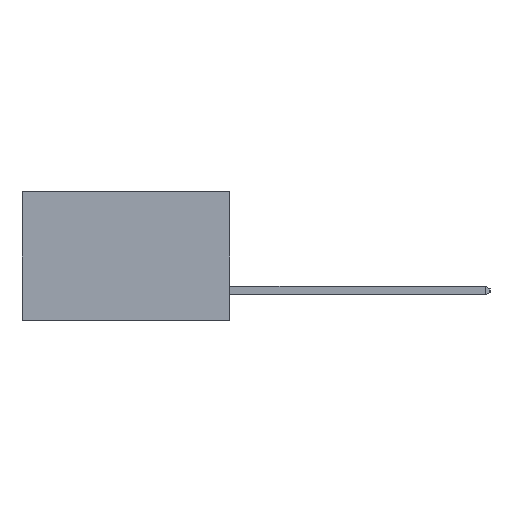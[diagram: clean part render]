
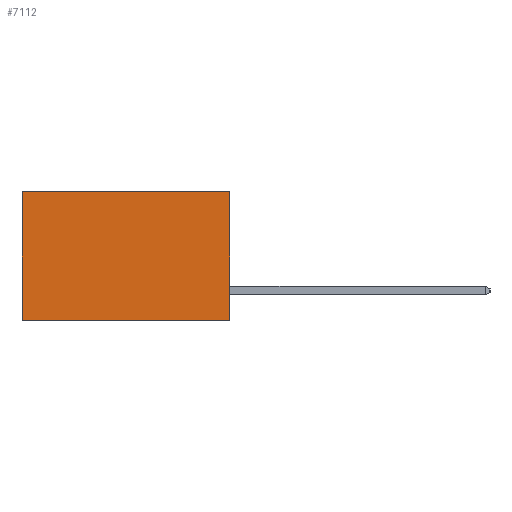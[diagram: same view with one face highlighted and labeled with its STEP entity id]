
A CAD part, left-side view. The second image highlights one B-rep face of the part: STEP entity #7112.
In plain terms, the highlighted planar face has unit normal (-1, 0, 0).
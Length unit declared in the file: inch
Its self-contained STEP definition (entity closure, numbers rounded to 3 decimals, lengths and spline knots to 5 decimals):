
#264 = VERTEX_POINT ( 'NONE', #8954 ) ;
#1245 = CARTESIAN_POINT ( 'NONE',  ( 0.2615, 0., -0.37 ) ) ;
#1441 = CARTESIAN_POINT ( 'NONE',  ( 0.2615, 0.6, -0.37 ) ) ;
#2719 = ORIENTED_EDGE ( 'NONE', *, *, #11743, .F. ) ;
#3245 = AXIS2_PLACEMENT_3D ( 'NONE', #10856, #10905, #10511 ) ;
#3385 = FACE_OUTER_BOUND ( 'NONE', #14714, .T. ) ;
#4093 = CARTESIAN_POINT ( 'NONE',  ( 0.2615, 0.6, 0. ) ) ;
#4320 = VERTEX_POINT ( 'NONE', #4093 ) ;
#4349 = VECTOR ( 'NONE', #14608, 39.37008 ) ;
#4950 = EDGE_CURVE ( 'NONE', #4320, #10827, #7519, .T. ) ;
#5861 = VECTOR ( 'NONE', #13025, 39.37008 ) ;
#6840 = DIRECTION ( 'NONE',  ( 0., 1., 0. ) ) ;
#6980 = LINE ( 'NONE', #12614, #13125 ) ;
#7112 = ADVANCED_FACE ( 'NONE', ( #3385 ), #12283, .F. ) ;
#7519 = LINE ( 'NONE', #14672, #4349 ) ;
#8954 = CARTESIAN_POINT ( 'NONE',  ( 0.2615, 0., -0.37 ) ) ;
#9126 = LINE ( 'NONE', #13814, #11797 ) ;
#9209 = EDGE_CURVE ( 'NONE', #10814, #264, #9126, .T. ) ;
#9389 = ORIENTED_EDGE ( 'NONE', *, *, #4950, .T. ) ;
#10349 = ORIENTED_EDGE ( 'NONE', *, *, #11684, .T. ) ;
#10511 = DIRECTION ( 'NONE',  ( 0., 0., -1. ) ) ;
#10626 = ORIENTED_EDGE ( 'NONE', *, *, #9209, .F. ) ;
#10814 = VERTEX_POINT ( 'NONE', #10917 ) ;
#10827 = VERTEX_POINT ( 'NONE', #1441 ) ;
#10856 = CARTESIAN_POINT ( 'NONE',  ( 0.2615, 0., -0.37 ) ) ;
#10905 = DIRECTION ( 'NONE',  ( 1., 0., 0. ) ) ;
#10917 = CARTESIAN_POINT ( 'NONE',  ( 0.2615, 0., 0. ) ) ;
#11684 = EDGE_CURVE ( 'NONE', #10814, #4320, #6980, .T. ) ;
#11743 = EDGE_CURVE ( 'NONE', #264, #10827, #12067, .T. ) ;
#11797 = VECTOR ( 'NONE', #14881, 39.37008 ) ;
#12067 = LINE ( 'NONE', #1245, #5861 ) ;
#12283 = PLANE ( 'NONE',  #3245 ) ;
#12614 = CARTESIAN_POINT ( 'NONE',  ( 0.2615, 0., 0. ) ) ;
#13025 = DIRECTION ( 'NONE',  ( 0., 1., 0. ) ) ;
#13125 = VECTOR ( 'NONE', #6840, 39.37008 ) ;
#13814 = CARTESIAN_POINT ( 'NONE',  ( 0.2615, 0., -0.37 ) ) ;
#14608 = DIRECTION ( 'NONE',  ( 0., 0., -1. ) ) ;
#14672 = CARTESIAN_POINT ( 'NONE',  ( 0.2615, 0.6, -0.37 ) ) ;
#14714 = EDGE_LOOP ( 'NONE', ( #9389, #2719, #10626, #10349 ) ) ;
#14881 = DIRECTION ( 'NONE',  ( 0., 0., -1. ) ) ;
